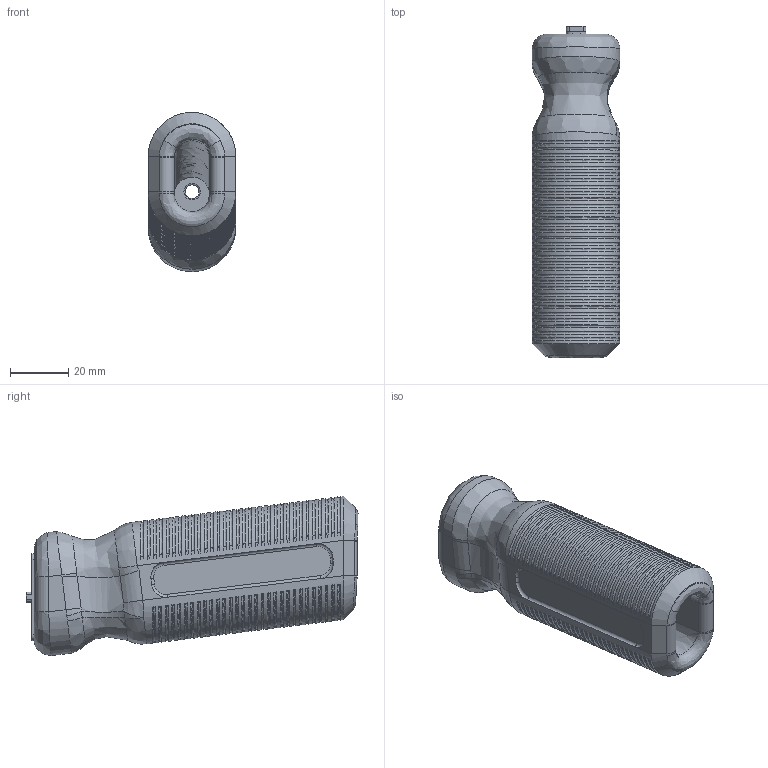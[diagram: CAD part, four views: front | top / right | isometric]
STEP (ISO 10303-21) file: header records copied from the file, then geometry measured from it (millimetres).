
FILE_DESCRIPTION(/* description */ (''),/* implementation_level */ '2;1');
FILE_NAME(/* name */ 'foregrip-mlok-freeman1337.step',/* time_stamp */ '2021-04-05T12:09:24-07:00',/* author */ (''),/* organization */ (''),/* preprocessor_version */ 'ST-DEVELOPER v18.1',/* originating_system */ 'Autodesk Translation Framework v9.10.0.1330',/* authorisation */ '');
FILE_SCHEMA (('AUTOMOTIVE_DESIGN { 1 0 10303 214 3 1 1 }'));
Length unit declared in the file: millimetre
Products named in the file (1): foregrip-mlok
Bounding box: 30 x 113.72 x 54.62 mm (x, y, z)
Volume: 80340.9 mm3; surface area: 22392 mm2
Topology: 1 solids, 1 shells, 511 faces, 1294 edges, 788 vertices
Faces by surface type: cylinder 218, bspline 190, plane 87, torus 16
Full cylindrical faces by diameter (mm): 4.65 x2
Entity records: 29128 total; most frequent: CARTESIAN_POINT 19010, ORIENTED_EDGE 2468, DIRECTION 1340, EDGE_CURVE 1234, VERTEX_POINT 788, B_SPLINE_CURVE_WITH_KNOTS 712, EDGE_LOOP 578, FACE_OUTER_BOUND 511
